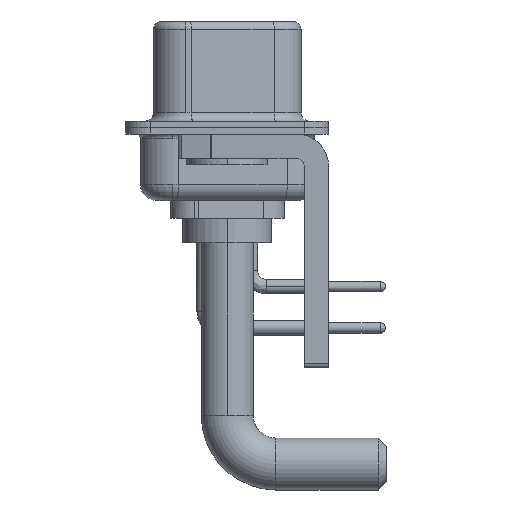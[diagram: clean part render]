
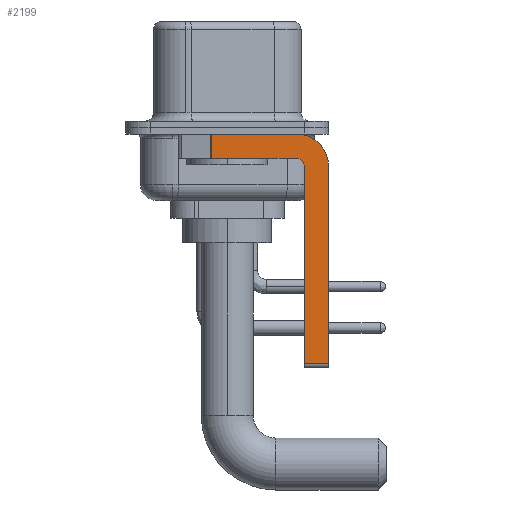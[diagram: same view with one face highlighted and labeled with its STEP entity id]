
A CAD part, left-side view. The second image highlights one B-rep face of the part: STEP entity #2199.
In plain terms, the highlighted planar face has unit normal (-1, 0, 0).
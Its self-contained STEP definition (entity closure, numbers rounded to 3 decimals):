
#95 = EDGE_CURVE ( 'NONE', #14720, #9429, #25752, .T. ) ;
#475 = EDGE_CURVE ( 'NONE', #10989, #10632, #17559, .T. ) ;
#745 = CARTESIAN_POINT ( 'NONE',  ( -2.9, -4.25, -2.4 ) ) ;
#1238 = EDGE_CURVE ( 'NONE', #10632, #6452, #16768, .T. ) ;
#1359 = VECTOR ( 'NONE', #2084, 1000. ) ;
#1528 = CARTESIAN_POINT ( 'NONE',  ( -2.9, -4.25, -2.4 ) ) ;
#2084 = DIRECTION ( 'NONE',  ( 0., 0., 1. ) ) ;
#2199 = ADVANCED_FACE ( 'NONE', ( #8616 ), #4642, .F. ) ;
#2609 = LINE ( 'NONE', #10740, #16254 ) ;
#2742 = DIRECTION ( 'NONE',  ( 1., 0., 0. ) ) ;
#4642 = PLANE ( 'NONE',  #16401 ) ;
#5182 = CARTESIAN_POINT ( 'NONE',  ( -2.9, 3., -0.4 ) ) ;
#6075 = DIRECTION ( 'NONE',  ( 0., 0., -1. ) ) ;
#6104 = CARTESIAN_POINT ( 'NONE',  ( -2.9, -4.75, -14.8 ) ) ;
#6452 = VERTEX_POINT ( 'NONE', #14119 ) ;
#6546 = VERTEX_POINT ( 'NONE', #8991 ) ;
#6982 = AXIS2_PLACEMENT_3D ( 'NONE', #16742, #23780, #16169 ) ;
#7471 = DIRECTION ( 'NONE',  ( 0., 1., 0. ) ) ;
#7875 = ORIENTED_EDGE ( 'NONE', *, *, #25929, .F. ) ;
#8002 = CARTESIAN_POINT ( 'NONE',  ( -2.9, 0.978, -0.4 ) ) ;
#8433 = DIRECTION ( 'NONE',  ( 0., 0., -1. ) ) ;
#8553 = LINE ( 'NONE', #16552, #8977 ) ;
#8616 = FACE_OUTER_BOUND ( 'NONE', #12963, .T. ) ;
#8936 = ORIENTED_EDGE ( 'NONE', *, *, #10507, .T. ) ;
#8977 = VECTOR ( 'NONE', #8433, 1000. ) ;
#8991 = CARTESIAN_POINT ( 'NONE',  ( -2.9, -4.75, -14.55 ) ) ;
#9429 = VERTEX_POINT ( 'NONE', #15305 ) ;
#9507 = CARTESIAN_POINT ( 'NONE',  ( -2.9, -6.25, -14.55 ) ) ;
#9510 = CIRCLE ( 'NONE', #6982, 0.5 ) ;
#9594 = CARTESIAN_POINT ( 'NONE',  ( -2.9, -4.25, -1.9 ) ) ;
#10507 = EDGE_CURVE ( 'NONE', #10989, #9429, #8553, .T. ) ;
#10632 = VERTEX_POINT ( 'NONE', #13335 ) ;
#10740 = CARTESIAN_POINT ( 'NONE',  ( -2.9, -6.25, -2.4 ) ) ;
#10989 = VERTEX_POINT ( 'NONE', #8002 ) ;
#11151 = VECTOR ( 'NONE', #7471, 1000. ) ;
#11494 = EDGE_CURVE ( 'NONE', #6452, #14056, #2609, .T. ) ;
#12337 = ORIENTED_EDGE ( 'NONE', *, *, #1238, .F. ) ;
#12887 = VECTOR ( 'NONE', #13568, 1000. ) ;
#12963 = EDGE_LOOP ( 'NONE', ( #16598, #8936, #22931, #7875, #22657, #13992, #20465, #12337 ) ) ;
#13335 = CARTESIAN_POINT ( 'NONE',  ( -2.9, -4.25, -0.4 ) ) ;
#13568 = DIRECTION ( 'NONE',  ( 0., -1., 0. ) ) ;
#13606 = LINE ( 'NONE', #21607, #18617 ) ;
#13992 = ORIENTED_EDGE ( 'NONE', *, *, #18290, .T. ) ;
#14056 = VERTEX_POINT ( 'NONE', #9507 ) ;
#14119 = CARTESIAN_POINT ( 'NONE',  ( -2.9, -6.25, -2.4 ) ) ;
#14720 = VERTEX_POINT ( 'NONE', #24417 ) ;
#14750 = DIRECTION ( 'NONE',  ( 0., 0., -1. ) ) ;
#14878 = DIRECTION ( 'NONE',  ( 0., 0., -1. ) ) ;
#15305 = CARTESIAN_POINT ( 'NONE',  ( -2.9, 0.978, -1.9 ) ) ;
#15902 = VERTEX_POINT ( 'NONE', #21954 ) ;
#16169 = DIRECTION ( 'NONE',  ( 0., 0., 1. ) ) ;
#16254 = VECTOR ( 'NONE', #14750, 1000. ) ;
#16401 = AXIS2_PLACEMENT_3D ( 'NONE', #745, #2742, #14878 ) ;
#16552 = CARTESIAN_POINT ( 'NONE',  ( -2.9, 0.978, -1.9 ) ) ;
#16598 = ORIENTED_EDGE ( 'NONE', *, *, #475, .F. ) ;
#16742 = CARTESIAN_POINT ( 'NONE',  ( -2.9, -4.25, -2.4 ) ) ;
#16768 = CIRCLE ( 'NONE', #23171, 2. ) ;
#17559 = LINE ( 'NONE', #5182, #12887 ) ;
#18290 = EDGE_CURVE ( 'NONE', #6546, #14056, #13606, .T. ) ;
#18617 = VECTOR ( 'NONE', #23866, 1000. ) ;
#20465 = ORIENTED_EDGE ( 'NONE', *, *, #11494, .F. ) ;
#21607 = CARTESIAN_POINT ( 'NONE',  ( -2.9, -4.25, -14.55 ) ) ;
#21954 = CARTESIAN_POINT ( 'NONE',  ( -2.9, -4.75, -2.4 ) ) ;
#22657 = ORIENTED_EDGE ( 'NONE', *, *, #22817, .F. ) ;
#22817 = EDGE_CURVE ( 'NONE', #6546, #15902, #24350, .T. ) ;
#22931 = ORIENTED_EDGE ( 'NONE', *, *, #95, .F. ) ;
#23171 = AXIS2_PLACEMENT_3D ( 'NONE', #1528, #24069, #6075 ) ;
#23780 = DIRECTION ( 'NONE',  ( -1., 0., 0. ) ) ;
#23866 = DIRECTION ( 'NONE',  ( 0., -1., 0. ) ) ;
#24069 = DIRECTION ( 'NONE',  ( 1., 0., 0. ) ) ;
#24350 = LINE ( 'NONE', #6104, #1359 ) ;
#24417 = CARTESIAN_POINT ( 'NONE',  ( -2.9, -4.25, -1.9 ) ) ;
#25752 = LINE ( 'NONE', #9594, #11151 ) ;
#25929 = EDGE_CURVE ( 'NONE', #15902, #14720, #9510, .T. ) ;
